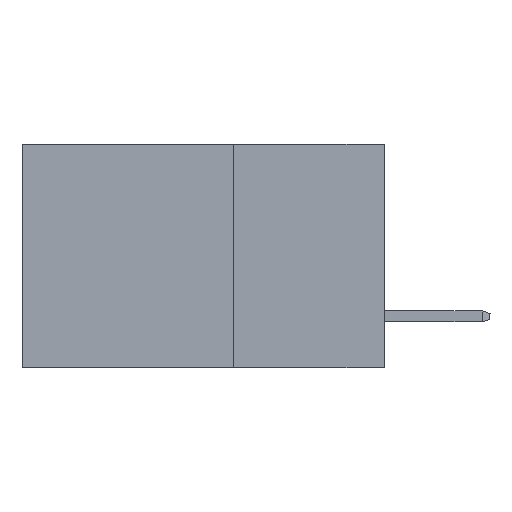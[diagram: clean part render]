
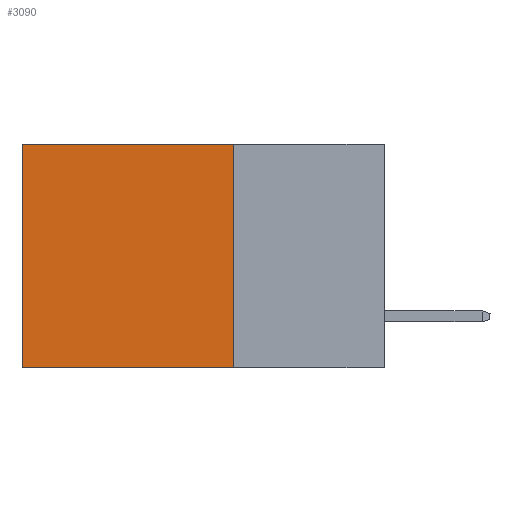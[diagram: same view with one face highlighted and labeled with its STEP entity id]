
A CAD part, left-side view. The second image highlights one B-rep face of the part: STEP entity #3090.
In plain terms, the highlighted planar face has unit normal (-1, 0, 0).
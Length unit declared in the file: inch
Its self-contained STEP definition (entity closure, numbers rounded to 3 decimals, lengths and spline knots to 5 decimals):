
#714 = CARTESIAN_POINT ( 'NONE',  ( 0.2615, 0.25, 0. ) ) ;
#859 = CARTESIAN_POINT ( 'NONE',  ( 0.2615, 0.25, -0.37 ) ) ;
#1079 = VERTEX_POINT ( 'NONE', #3355 ) ;
#1269 = VERTEX_POINT ( 'NONE', #17306 ) ;
#1498 = DIRECTION ( 'NONE',  ( 0., 0., -1. ) ) ;
#1587 = EDGE_CURVE ( 'NONE', #5531, #14917, #16074, .T. ) ;
#3090 = ADVANCED_FACE ( 'NONE', ( #21255 ), #6055, .F. ) ;
#3355 = CARTESIAN_POINT ( 'NONE',  ( 0.2615, 0.6, -0.37 ) ) ;
#3978 = LINE ( 'NONE', #16098, #5268 ) ;
#4726 = DIRECTION ( 'NONE',  ( 1., 0., 0. ) ) ;
#4834 = LINE ( 'NONE', #11293, #10145 ) ;
#5268 = VECTOR ( 'NONE', #9005, 39.37008 ) ;
#5531 = VERTEX_POINT ( 'NONE', #714 ) ;
#6055 = PLANE ( 'NONE',  #17389 ) ;
#6305 = VECTOR ( 'NONE', #21821, 39.37008 ) ;
#6494 = EDGE_CURVE ( 'NONE', #5531, #1269, #3978, .T. ) ;
#7773 = CARTESIAN_POINT ( 'NONE',  ( 0.2615, 0.25, -0.37 ) ) ;
#7792 = VECTOR ( 'NONE', #14871, 39.37008 ) ;
#7795 = ORIENTED_EDGE ( 'NONE', *, *, #6494, .T. ) ;
#9005 = DIRECTION ( 'NONE',  ( 0., 1., 0. ) ) ;
#9323 = EDGE_CURVE ( 'NONE', #14917, #1079, #16818, .T. ) ;
#9731 = DIRECTION ( 'NONE',  ( 0., 0., -1. ) ) ;
#10145 = VECTOR ( 'NONE', #1498, 39.37008 ) ;
#11293 = CARTESIAN_POINT ( 'NONE',  ( 0.2615, 0.6, -0.37 ) ) ;
#13203 = CARTESIAN_POINT ( 'NONE',  ( 0.2615, 0.25, -0.37 ) ) ;
#14355 = ORIENTED_EDGE ( 'NONE', *, *, #9323, .F. ) ;
#14418 = EDGE_LOOP ( 'NONE', ( #18038, #14355, #20737, #7795 ) ) ;
#14871 = DIRECTION ( 'NONE',  ( 0., 1., 0. ) ) ;
#14917 = VERTEX_POINT ( 'NONE', #7773 ) ;
#16074 = LINE ( 'NONE', #859, #6305 ) ;
#16098 = CARTESIAN_POINT ( 'NONE',  ( 0.2615, 0.25, 0. ) ) ;
#16818 = LINE ( 'NONE', #21713, #7792 ) ;
#17306 = CARTESIAN_POINT ( 'NONE',  ( 0.2615, 0.6, 0. ) ) ;
#17389 = AXIS2_PLACEMENT_3D ( 'NONE', #13203, #4726, #9731 ) ;
#18013 = EDGE_CURVE ( 'NONE', #1269, #1079, #4834, .T. ) ;
#18038 = ORIENTED_EDGE ( 'NONE', *, *, #18013, .T. ) ;
#20737 = ORIENTED_EDGE ( 'NONE', *, *, #1587, .F. ) ;
#21255 = FACE_OUTER_BOUND ( 'NONE', #14418, .T. ) ;
#21713 = CARTESIAN_POINT ( 'NONE',  ( 0.2615, 0.25, -0.37 ) ) ;
#21821 = DIRECTION ( 'NONE',  ( 0., 0., -1. ) ) ;
